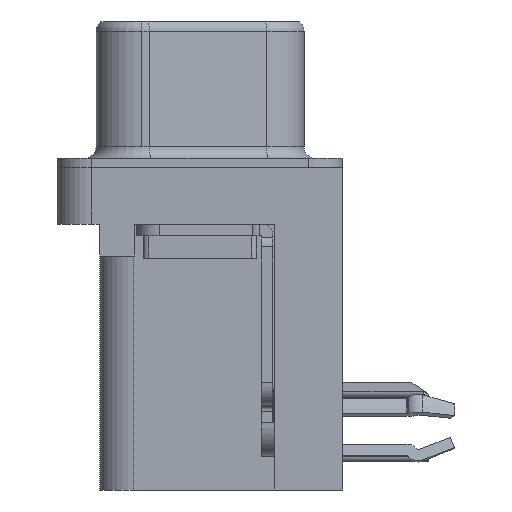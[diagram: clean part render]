
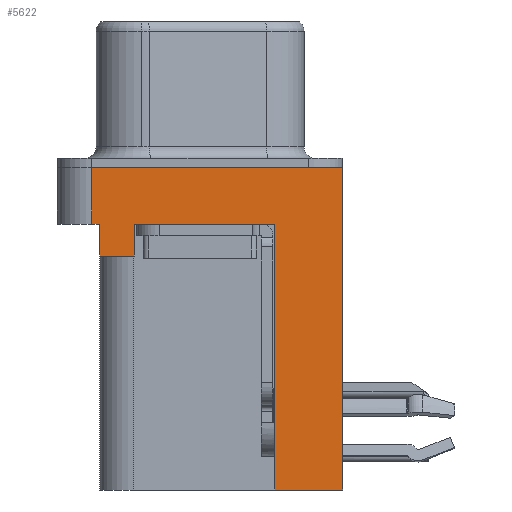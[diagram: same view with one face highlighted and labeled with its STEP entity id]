
A CAD part, left-side view. The second image highlights one B-rep face of the part: STEP entity #5622.
In plain terms, the highlighted planar face has unit normal (-1, 0, 0).
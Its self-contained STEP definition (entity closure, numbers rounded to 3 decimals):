
#38 = EDGE_CURVE ( 'NONE', #8733, #13087, #9636, .T. ) ;
#39 = CARTESIAN_POINT ( 'NONE',  ( -2.91, -3.295, -14.2 ) ) ;
#132 = VECTOR ( 'NONE', #14299, 1000. ) ;
#313 = VERTEX_POINT ( 'NONE', #12863 ) ;
#597 = ORIENTED_EDGE ( 'NONE', *, *, #15030, .F. ) ;
#672 = VECTOR ( 'NONE', #17609, 1000. ) ;
#1473 = CARTESIAN_POINT ( 'NONE',  ( -2.91, 4.425, -3.9 ) ) ;
#1553 = DIRECTION ( 'NONE',  ( 0., 0., 1. ) ) ;
#1924 = CARTESIAN_POINT ( 'NONE',  ( -2.91, 4.775, -2.5 ) ) ;
#1987 = VERTEX_POINT ( 'NONE', #14819 ) ;
#2359 = CARTESIAN_POINT ( 'NONE',  ( -2.91, -6.275, -2.5 ) ) ;
#2361 = CARTESIAN_POINT ( 'NONE',  ( -2.91, 4.775, 0. ) ) ;
#2532 = DIRECTION ( 'NONE',  ( 0., 0., 1. ) ) ;
#2947 = ORIENTED_EDGE ( 'NONE', *, *, #6117, .T. ) ;
#2953 = CARTESIAN_POINT ( 'NONE',  ( -2.91, -3.295, -14.2 ) ) ;
#3691 = VERTEX_POINT ( 'NONE', #15410 ) ;
#3787 = ORIENTED_EDGE ( 'NONE', *, *, #13468, .F. ) ;
#3795 = CARTESIAN_POINT ( 'NONE',  ( -2.91, -3.295, -2.5 ) ) ;
#3830 = DIRECTION ( 'NONE',  ( -1., 0., 0. ) ) ;
#4394 = VECTOR ( 'NONE', #7333, 1000. ) ;
#4527 = VECTOR ( 'NONE', #16807, 1000. ) ;
#4772 = VECTOR ( 'NONE', #7840, 1000. ) ;
#4997 = VERTEX_POINT ( 'NONE', #12577 ) ;
#5059 = LINE ( 'NONE', #2359, #4772 ) ;
#5302 = CARTESIAN_POINT ( 'NONE',  ( -2.91, 2.895, -2.5 ) ) ;
#5402 = EDGE_CURVE ( 'NONE', #7972, #14022, #5726, .T. ) ;
#5571 = EDGE_CURVE ( 'NONE', #9259, #7972, #6690, .T. ) ;
#5622 = ADVANCED_FACE ( 'NONE', ( #17700 ), #6870, .T. ) ;
#5726 = LINE ( 'NONE', #8603, #4394 ) ;
#5795 = DIRECTION ( 'NONE',  ( 0., 0., 1. ) ) ;
#6117 = EDGE_CURVE ( 'NONE', #8733, #4997, #5059, .T. ) ;
#6690 = LINE ( 'NONE', #16353, #672 ) ;
#6870 = PLANE ( 'NONE',  #7563 ) ;
#7333 = DIRECTION ( 'NONE',  ( 0., -1., 0. ) ) ;
#7518 = VERTEX_POINT ( 'NONE', #2361 ) ;
#7563 = AXIS2_PLACEMENT_3D ( 'NONE', #11986, #3830, #16270 ) ;
#7619 = ORIENTED_EDGE ( 'NONE', *, *, #5402, .T. ) ;
#7840 = DIRECTION ( 'NONE',  ( 0., 0., 1. ) ) ;
#7972 = VERTEX_POINT ( 'NONE', #5302 ) ;
#8095 = EDGE_CURVE ( 'NONE', #313, #1987, #8435, .T. ) ;
#8435 = LINE ( 'NONE', #16582, #16229 ) ;
#8603 = CARTESIAN_POINT ( 'NONE',  ( -2.91, -6.275, -2.5 ) ) ;
#8733 = VERTEX_POINT ( 'NONE', #15238 ) ;
#8841 = LINE ( 'NONE', #15892, #132 ) ;
#9259 = VERTEX_POINT ( 'NONE', #16829 ) ;
#9271 = LINE ( 'NONE', #9358, #13427 ) ;
#9358 = CARTESIAN_POINT ( 'NONE',  ( -2.91, -3.295, -14.2 ) ) ;
#9636 = LINE ( 'NONE', #39, #16774 ) ;
#10181 = CARTESIAN_POINT ( 'NONE',  ( -2.91, 4.425, -3.9 ) ) ;
#10723 = DIRECTION ( 'NONE',  ( 0., 1., 0. ) ) ;
#10825 = VECTOR ( 'NONE', #5795, 1000. ) ;
#10876 = EDGE_CURVE ( 'NONE', #7518, #4997, #8841, .T. ) ;
#11986 = CARTESIAN_POINT ( 'NONE',  ( -2.91, -6.275, -2.5 ) ) ;
#12577 = CARTESIAN_POINT ( 'NONE',  ( -2.91, -6.275, 0. ) ) ;
#12863 = CARTESIAN_POINT ( 'NONE',  ( -2.91, 4.775, -2.5 ) ) ;
#13087 = VERTEX_POINT ( 'NONE', #2953 ) ;
#13126 = VECTOR ( 'NONE', #1553, 1000. ) ;
#13427 = VECTOR ( 'NONE', #2532, 1000. ) ;
#13446 = EDGE_CURVE ( 'NONE', #9259, #3691, #16713, .T. ) ;
#13468 = EDGE_CURVE ( 'NONE', #313, #7518, #17074, .T. ) ;
#13496 = ORIENTED_EDGE ( 'NONE', *, *, #38, .F. ) ;
#13501 = LINE ( 'NONE', #1473, #13126 ) ;
#14022 = VERTEX_POINT ( 'NONE', #3795 ) ;
#14287 = ORIENTED_EDGE ( 'NONE', *, *, #13446, .F. ) ;
#14299 = DIRECTION ( 'NONE',  ( 0., -1., 0. ) ) ;
#14352 = ORIENTED_EDGE ( 'NONE', *, *, #5571, .T. ) ;
#14713 = ORIENTED_EDGE ( 'NONE', *, *, #8095, .T. ) ;
#14819 = CARTESIAN_POINT ( 'NONE',  ( -2.91, 4.425, -2.5 ) ) ;
#14970 = DIRECTION ( 'NONE',  ( 0., -1., 0. ) ) ;
#14986 = ORIENTED_EDGE ( 'NONE', *, *, #10876, .F. ) ;
#15030 = EDGE_CURVE ( 'NONE', #13087, #14022, #9271, .T. ) ;
#15238 = CARTESIAN_POINT ( 'NONE',  ( -2.91, -6.275, -14.2 ) ) ;
#15410 = CARTESIAN_POINT ( 'NONE',  ( -2.91, 4.425, -3.9 ) ) ;
#15802 = EDGE_CURVE ( 'NONE', #3691, #1987, #13501, .T. ) ;
#15892 = CARTESIAN_POINT ( 'NONE',  ( -2.91, -6.275, 0. ) ) ;
#16076 = ORIENTED_EDGE ( 'NONE', *, *, #15802, .F. ) ;
#16229 = VECTOR ( 'NONE', #14970, 1000. ) ;
#16253 = EDGE_LOOP ( 'NONE', ( #14986, #3787, #14713, #16076, #14287, #14352, #7619, #597, #13496, #2947 ) ) ;
#16270 = DIRECTION ( 'NONE',  ( 0., 0., 1. ) ) ;
#16353 = CARTESIAN_POINT ( 'NONE',  ( -2.91, 2.895, -3.9 ) ) ;
#16582 = CARTESIAN_POINT ( 'NONE',  ( -2.91, -6.275, -2.5 ) ) ;
#16713 = LINE ( 'NONE', #10181, #4527 ) ;
#16774 = VECTOR ( 'NONE', #10723, 1000. ) ;
#16807 = DIRECTION ( 'NONE',  ( 0., 1., 0. ) ) ;
#16829 = CARTESIAN_POINT ( 'NONE',  ( -2.91, 2.895, -3.9 ) ) ;
#17074 = LINE ( 'NONE', #1924, #10825 ) ;
#17609 = DIRECTION ( 'NONE',  ( 0., 0., 1. ) ) ;
#17700 = FACE_OUTER_BOUND ( 'NONE', #16253, .T. ) ;
